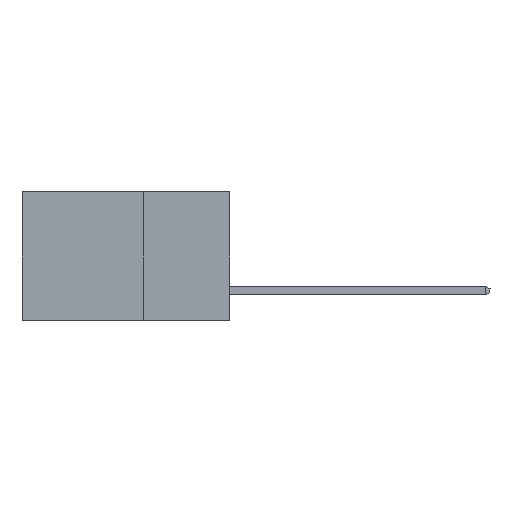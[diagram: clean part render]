
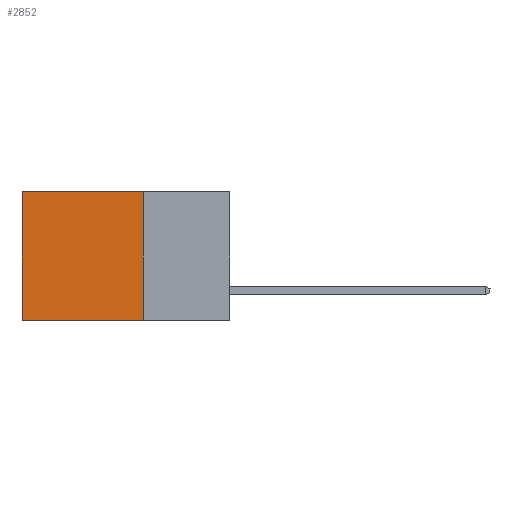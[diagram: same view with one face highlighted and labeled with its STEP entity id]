
A CAD part, left-side view. The second image highlights one B-rep face of the part: STEP entity #2852.
In plain terms, the highlighted planar face has unit normal (-1, 0, 0).
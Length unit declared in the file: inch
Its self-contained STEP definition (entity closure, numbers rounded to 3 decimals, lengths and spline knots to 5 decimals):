
#91 = AXIS2_PLACEMENT_3D ( 'NONE', #17396, #1759, #4016 ) ;
#348 = DIRECTION ( 'NONE',  ( 0., 1., 0. ) ) ;
#698 = VECTOR ( 'NONE', #17452, 39.37008 ) ;
#832 = LINE ( 'NONE', #20221, #7791 ) ;
#882 = VECTOR ( 'NONE', #22358, 39.37008 ) ;
#1580 = VECTOR ( 'NONE', #348, 39.37008 ) ;
#1703 = LINE ( 'NONE', #8672, #698 ) ;
#1759 = DIRECTION ( 'NONE',  ( 1., 0., 0. ) ) ;
#2321 = VERTEX_POINT ( 'NONE', #10904 ) ;
#2852 = ADVANCED_FACE ( 'NONE', ( #20814 ), #21038, .F. ) ;
#4016 = DIRECTION ( 'NONE',  ( 0., 0., -1. ) ) ;
#4595 = CARTESIAN_POINT ( 'NONE',  ( 0.2615, 0.25, 0. ) ) ;
#5955 = ORIENTED_EDGE ( 'NONE', *, *, #17532, .F. ) ;
#6990 = VERTEX_POINT ( 'NONE', #4595 ) ;
#7791 = VECTOR ( 'NONE', #8244, 39.37008 ) ;
#8244 = DIRECTION ( 'NONE',  ( 0., 1., 0. ) ) ;
#8672 = CARTESIAN_POINT ( 'NONE',  ( 0.2615, 0.6, -0.37 ) ) ;
#10163 = EDGE_CURVE ( 'NONE', #14707, #2321, #1703, .T. ) ;
#10271 = CARTESIAN_POINT ( 'NONE',  ( 0.2615, 0.25, -0.37 ) ) ;
#10746 = LINE ( 'NONE', #17708, #1580 ) ;
#10904 = CARTESIAN_POINT ( 'NONE',  ( 0.2615, 0.6, -0.37 ) ) ;
#11246 = ORIENTED_EDGE ( 'NONE', *, *, #10163, .T. ) ;
#11759 = CARTESIAN_POINT ( 'NONE',  ( 0.2615, 0.25, -0.37 ) ) ;
#12423 = ORIENTED_EDGE ( 'NONE', *, *, #14773, .T. ) ;
#14707 = VERTEX_POINT ( 'NONE', #17821 ) ;
#14773 = EDGE_CURVE ( 'NONE', #6990, #14707, #10746, .T. ) ;
#15416 = LINE ( 'NONE', #11759, #882 ) ;
#16897 = EDGE_CURVE ( 'NONE', #17464, #2321, #832, .T. ) ;
#17396 = CARTESIAN_POINT ( 'NONE',  ( 0.2615, 0.25, -0.37 ) ) ;
#17452 = DIRECTION ( 'NONE',  ( 0., 0., -1. ) ) ;
#17464 = VERTEX_POINT ( 'NONE', #10271 ) ;
#17532 = EDGE_CURVE ( 'NONE', #6990, #17464, #15416, .T. ) ;
#17708 = CARTESIAN_POINT ( 'NONE',  ( 0.2615, 0.25, 0. ) ) ;
#17821 = CARTESIAN_POINT ( 'NONE',  ( 0.2615, 0.6, 0. ) ) ;
#19019 = ORIENTED_EDGE ( 'NONE', *, *, #16897, .F. ) ;
#20221 = CARTESIAN_POINT ( 'NONE',  ( 0.2615, 0.25, -0.37 ) ) ;
#20814 = FACE_OUTER_BOUND ( 'NONE', #21667, .T. ) ;
#21038 = PLANE ( 'NONE',  #91 ) ;
#21667 = EDGE_LOOP ( 'NONE', ( #11246, #19019, #5955, #12423 ) ) ;
#22358 = DIRECTION ( 'NONE',  ( 0., 0., -1. ) ) ;
